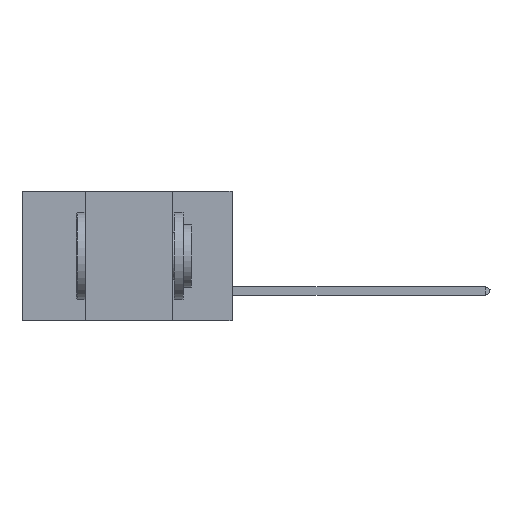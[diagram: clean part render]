
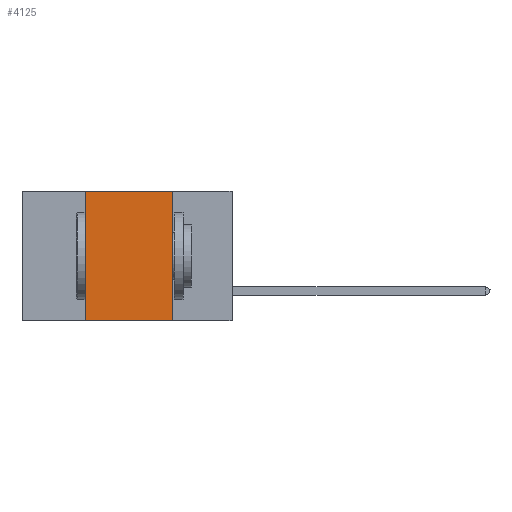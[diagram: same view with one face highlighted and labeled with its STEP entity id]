
A CAD part, left-side view. The second image highlights one B-rep face of the part: STEP entity #4125.
In plain terms, the highlighted planar face has unit normal (-1, 0, 0).
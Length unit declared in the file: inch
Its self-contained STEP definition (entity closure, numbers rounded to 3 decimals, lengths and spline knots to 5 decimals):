
#66 = EDGE_CURVE ( 'NONE', #19037, #24843, #17778, .T. ) ;
#496 = LINE ( 'NONE', #635, #5622 ) ;
#635 = CARTESIAN_POINT ( 'NONE',  ( 0., 0.17, 0. ) ) ;
#1162 = CARTESIAN_POINT ( 'NONE',  ( 0., 0.6, 0. ) ) ;
#1808 = EDGE_CURVE ( 'NONE', #2348, #4345, #3195, .T. ) ;
#2131 = CARTESIAN_POINT ( 'NONE',  ( 0., 0.42, -0.37 ) ) ;
#2348 = VERTEX_POINT ( 'NONE', #2131 ) ;
#2552 = DIRECTION ( 'NONE',  ( 0., 0., -1. ) ) ;
#3195 = LINE ( 'NONE', #13216, #21899 ) ;
#4125 = ADVANCED_FACE ( 'NONE', ( #24248 ), #8274, .F. ) ;
#4206 = ORIENTED_EDGE ( 'NONE', *, *, #17284, .F. ) ;
#4230 = CARTESIAN_POINT ( 'NONE',  ( 0., 0.17, 0. ) ) ;
#4345 = VERTEX_POINT ( 'NONE', #5125 ) ;
#5125 = CARTESIAN_POINT ( 'NONE',  ( 0., 0.17, -0.37 ) ) ;
#5622 = VECTOR ( 'NONE', #2552, 39.37008 ) ;
#6536 = ORIENTED_EDGE ( 'NONE', *, *, #24379, .F. ) ;
#8274 = PLANE ( 'NONE',  #20680 ) ;
#10940 = DIRECTION ( 'NONE',  ( 0., -1., 0. ) ) ;
#10983 = VECTOR ( 'NONE', #17074, 39.37008 ) ;
#13216 = CARTESIAN_POINT ( 'NONE',  ( 0., 0.6, -0.37 ) ) ;
#15020 = CARTESIAN_POINT ( 'NONE',  ( 0., 0.42, 0. ) ) ;
#15874 = ORIENTED_EDGE ( 'NONE', *, *, #1808, .T. ) ;
#16525 = DIRECTION ( 'NONE',  ( 1., 0., 0. ) ) ;
#17074 = DIRECTION ( 'NONE',  ( 0., 0., 1. ) ) ;
#17284 = EDGE_CURVE ( 'NONE', #2348, #19037, #22130, .T. ) ;
#17778 = LINE ( 'NONE', #24658, #19030 ) ;
#18155 = EDGE_LOOP ( 'NONE', ( #6536, #21951, #4206, #15874 ) ) ;
#18755 = CARTESIAN_POINT ( 'NONE',  ( 0., 0.42, 0. ) ) ;
#19030 = VECTOR ( 'NONE', #10940, 39.37008 ) ;
#19037 = VERTEX_POINT ( 'NONE', #15020 ) ;
#20680 = AXIS2_PLACEMENT_3D ( 'NONE', #1162, #16525, #22402 ) ;
#21899 = VECTOR ( 'NONE', #24647, 39.37008 ) ;
#21951 = ORIENTED_EDGE ( 'NONE', *, *, #66, .F. ) ;
#22130 = LINE ( 'NONE', #18755, #10983 ) ;
#22402 = DIRECTION ( 'NONE',  ( 0., 0., -1. ) ) ;
#24248 = FACE_OUTER_BOUND ( 'NONE', #18155, .T. ) ;
#24379 = EDGE_CURVE ( 'NONE', #24843, #4345, #496, .T. ) ;
#24647 = DIRECTION ( 'NONE',  ( 0., -1., 0. ) ) ;
#24658 = CARTESIAN_POINT ( 'NONE',  ( 0., 0.6, 0. ) ) ;
#24843 = VERTEX_POINT ( 'NONE', #4230 ) ;
